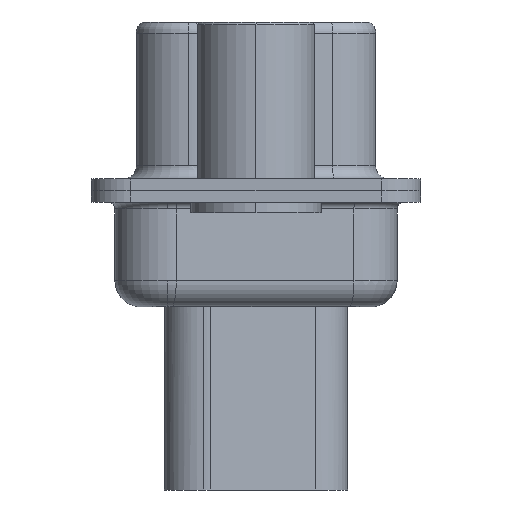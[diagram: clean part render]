
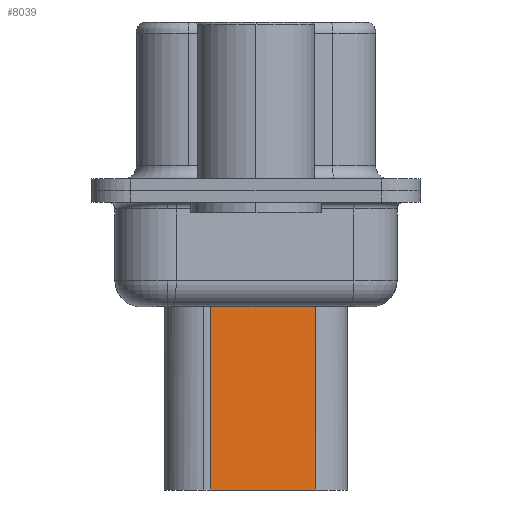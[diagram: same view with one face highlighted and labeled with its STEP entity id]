
A CAD part, left-side view. The second image highlights one B-rep face of the part: STEP entity #8039.
In plain terms, the highlighted planar face has unit normal (-0.985, -0.174, 0).
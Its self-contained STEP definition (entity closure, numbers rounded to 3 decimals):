
#208 = LINE ( 'NONE', #16858, #15299 ) ;
#222 = FACE_OUTER_BOUND ( 'NONE', #11777, .T. ) ;
#433 = VECTOR ( 'NONE', #7207, 1000. ) ;
#2192 = AXIS2_PLACEMENT_3D ( 'NONE', #8455, #18693, #9930 ) ;
#2558 = CARTESIAN_POINT ( 'NONE',  ( 5.229, -2.26, -3.1 ) ) ;
#3828 = VECTOR ( 'NONE', #6402, 1000. ) ;
#4849 = CARTESIAN_POINT ( 'NONE',  ( 5.229, -2.26, -11.45 ) ) ;
#4900 = ORIENTED_EDGE ( 'NONE', *, *, #12065, .F. ) ;
#5761 = CARTESIAN_POINT ( 'NONE',  ( 4.524, 1.74, -11.45 ) ) ;
#6402 = DIRECTION ( 'NONE',  ( -0.174, 0.985, 0. ) ) ;
#7207 = DIRECTION ( 'NONE',  ( -0.174, 0.985, 0. ) ) ;
#7706 = LINE ( 'NONE', #12202, #3828 ) ;
#8039 = ADVANCED_FACE ( 'NONE', ( #222 ), #15666, .T. ) ;
#8095 = DIRECTION ( 'NONE',  ( 0., 0., -1. ) ) ;
#8455 = CARTESIAN_POINT ( 'NONE',  ( 4.524, 1.74, -3.1 ) ) ;
#8651 = ORIENTED_EDGE ( 'NONE', *, *, #11798, .T. ) ;
#9500 = CARTESIAN_POINT ( 'NONE',  ( 5.229, -2.26, -3.975 ) ) ;
#9930 = DIRECTION ( 'NONE',  ( 0.174, -0.985, 0. ) ) ;
#10251 = EDGE_CURVE ( 'NONE', #18888, #12989, #7706, .T. ) ;
#10680 = VECTOR ( 'NONE', #11290, 1000. ) ;
#11290 = DIRECTION ( 'NONE',  ( 0., 0., -1. ) ) ;
#11777 = EDGE_LOOP ( 'NONE', ( #12471, #15633, #8651, #4900 ) ) ;
#11798 = EDGE_CURVE ( 'NONE', #12989, #16796, #208, .T. ) ;
#12065 = EDGE_CURVE ( 'NONE', #18420, #16796, #12121, .T. ) ;
#12121 = LINE ( 'NONE', #5761, #433 ) ;
#12202 = CARTESIAN_POINT ( 'NONE',  ( 4.353, 2.709, -3.975 ) ) ;
#12471 = ORIENTED_EDGE ( 'NONE', *, *, #17163, .F. ) ;
#12989 = VERTEX_POINT ( 'NONE', #13893 ) ;
#13502 = CARTESIAN_POINT ( 'NONE',  ( 4.524, 1.74, -11.45 ) ) ;
#13893 = CARTESIAN_POINT ( 'NONE',  ( 4.524, 1.74, -3.975 ) ) ;
#14126 = LINE ( 'NONE', #2558, #10680 ) ;
#15299 = VECTOR ( 'NONE', #8095, 1000. ) ;
#15633 = ORIENTED_EDGE ( 'NONE', *, *, #10251, .T. ) ;
#15666 = PLANE ( 'NONE',  #2192 ) ;
#16796 = VERTEX_POINT ( 'NONE', #13502 ) ;
#16858 = CARTESIAN_POINT ( 'NONE',  ( 4.524, 1.74, -3.1 ) ) ;
#17163 = EDGE_CURVE ( 'NONE', #18888, #18420, #14126, .T. ) ;
#18420 = VERTEX_POINT ( 'NONE', #4849 ) ;
#18693 = DIRECTION ( 'NONE',  ( -0.985, -0.174, 0. ) ) ;
#18888 = VERTEX_POINT ( 'NONE', #9500 ) ;
